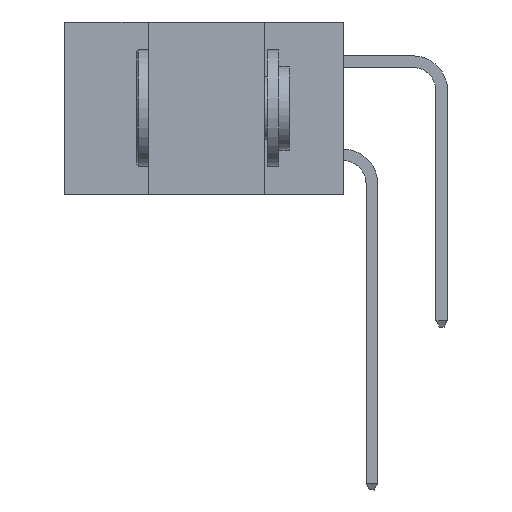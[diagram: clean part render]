
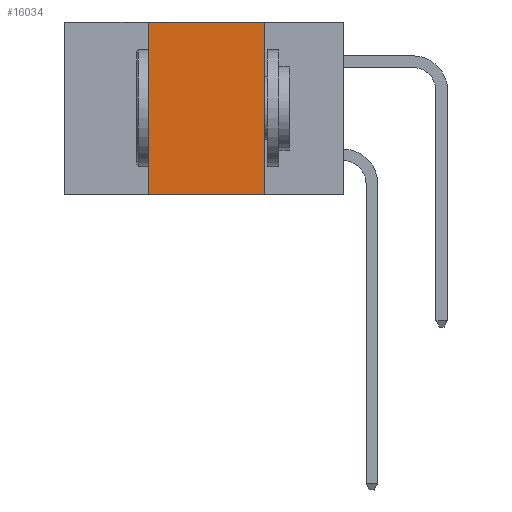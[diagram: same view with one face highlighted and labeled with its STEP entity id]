
A CAD part, left-side view. The second image highlights one B-rep face of the part: STEP entity #16034.
In plain terms, the highlighted planar face has unit normal (-1, 0, 0).
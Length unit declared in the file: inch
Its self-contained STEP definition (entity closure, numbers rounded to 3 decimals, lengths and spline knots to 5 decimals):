
#1238 = CARTESIAN_POINT ( 'NONE',  ( 0., 0.6, -0.37 ) ) ;
#2174 = CARTESIAN_POINT ( 'NONE',  ( 0., 0.42, 0. ) ) ;
#2348 = VERTEX_POINT ( 'NONE', #9038 ) ;
#3995 = VERTEX_POINT ( 'NONE', #19725 ) ;
#4008 = LINE ( 'NONE', #2174, #4646 ) ;
#4049 = CARTESIAN_POINT ( 'NONE',  ( 0., 0.17, -0.37 ) ) ;
#4646 = VECTOR ( 'NONE', #16333, 39.37008 ) ;
#4744 = EDGE_CURVE ( 'NONE', #2348, #13172, #5656, .T. ) ;
#5374 = LINE ( 'NONE', #10528, #20849 ) ;
#5656 = LINE ( 'NONE', #23957, #21132 ) ;
#5662 = CARTESIAN_POINT ( 'NONE',  ( 0., 0.42, 0. ) ) ;
#5672 = ORIENTED_EDGE ( 'NONE', *, *, #16870, .F. ) ;
#9038 = CARTESIAN_POINT ( 'NONE',  ( 0., 0.17, 0. ) ) ;
#10528 = CARTESIAN_POINT ( 'NONE',  ( 0., 0.6, 0. ) ) ;
#10606 = FACE_OUTER_BOUND ( 'NONE', #20442, .T. ) ;
#11226 = CARTESIAN_POINT ( 'NONE',  ( 0., 0.6, 0. ) ) ;
#11381 = DIRECTION ( 'NONE',  ( 0., -1., 0. ) ) ;
#12551 = DIRECTION ( 'NONE',  ( 0., -1., 0. ) ) ;
#12592 = DIRECTION ( 'NONE',  ( 0., 0., -1. ) ) ;
#13172 = VERTEX_POINT ( 'NONE', #4049 ) ;
#13250 = DIRECTION ( 'NONE',  ( 0., 0., -1. ) ) ;
#14736 = EDGE_CURVE ( 'NONE', #3995, #13172, #20204, .T. ) ;
#14794 = VECTOR ( 'NONE', #11381, 39.37008 ) ;
#16034 = ADVANCED_FACE ( 'NONE', ( #10606 ), #23324, .F. ) ;
#16333 = DIRECTION ( 'NONE',  ( 0., 0., 1. ) ) ;
#16870 = EDGE_CURVE ( 'NONE', #23991, #2348, #5374, .T. ) ;
#18945 = ORIENTED_EDGE ( 'NONE', *, *, #25495, .F. ) ;
#19725 = CARTESIAN_POINT ( 'NONE',  ( 0., 0.42, -0.37 ) ) ;
#19893 = ORIENTED_EDGE ( 'NONE', *, *, #4744, .F. ) ;
#19960 = AXIS2_PLACEMENT_3D ( 'NONE', #11226, #25324, #13250 ) ;
#20204 = LINE ( 'NONE', #1238, #14794 ) ;
#20442 = EDGE_LOOP ( 'NONE', ( #19893, #5672, #18945, #25517 ) ) ;
#20849 = VECTOR ( 'NONE', #12551, 39.37008 ) ;
#21132 = VECTOR ( 'NONE', #12592, 39.37008 ) ;
#23324 = PLANE ( 'NONE',  #19960 ) ;
#23957 = CARTESIAN_POINT ( 'NONE',  ( 0., 0.17, 0. ) ) ;
#23991 = VERTEX_POINT ( 'NONE', #5662 ) ;
#25324 = DIRECTION ( 'NONE',  ( 1., 0., 0. ) ) ;
#25495 = EDGE_CURVE ( 'NONE', #3995, #23991, #4008, .T. ) ;
#25517 = ORIENTED_EDGE ( 'NONE', *, *, #14736, .T. ) ;
